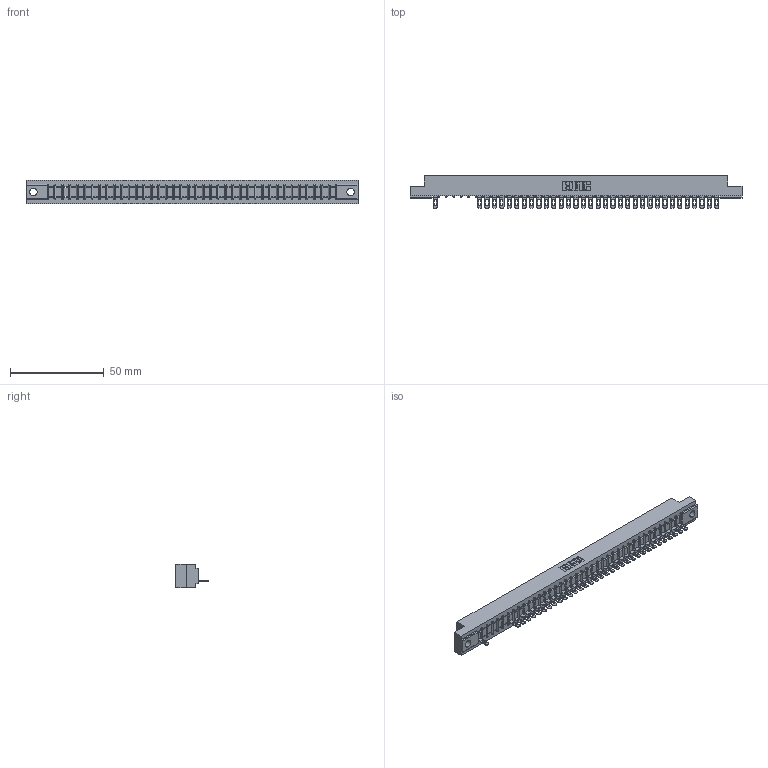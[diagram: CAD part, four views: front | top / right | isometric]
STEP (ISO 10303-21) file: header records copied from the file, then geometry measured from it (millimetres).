
FILE_DESCRIPTION (( 'STEP AP203' ), '1' );
FILE_NAME ('357-039-501-102.STEP', '2018-08-10T11:30:30', ( '' ), ( '' ), 'SwSTEP 2.0', 'SolidWorks 2016', '' );
FILE_SCHEMA (( 'CONFIG_CONTROL_DESIGN' ));
Length unit declared in the file: inch
Products named in the file (3): 307 Part_.128 Dia Mounting Holes; 307-290-002_501; 357-039-501-102
Assembly tree (35 placements, depth 2):
  357-039-501-102
    307 Part_.128 Dia Mounting Holes
    307-290-002_501  x34
Bounding box: 177.55 x 17.42 x 12.7 mm (x, y, z)
Volume: 18774.4 mm3; surface area: 22646.7 mm2
Topology: 35 solids, 35 shells, 2842 faces, 8735 edges, 5714 vertices
Faces by surface type: plane 1626, cylinder 1136, sphere 80
Entity records: 34440 total; most frequent: CARTESIAN_POINT 5831, ORIENTED_EDGE 5826, DIRECTION 5665, EDGE_CURVE 2913, VECTOR 2225, LINE 2225, VERTEX_POINT 1886, AXIS2_PLACEMENT_3D 1720
